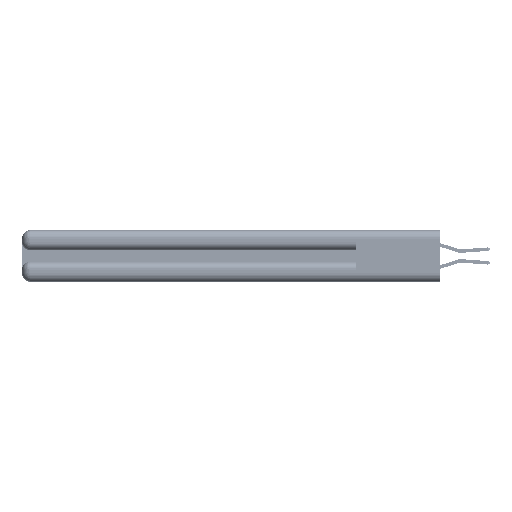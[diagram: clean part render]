
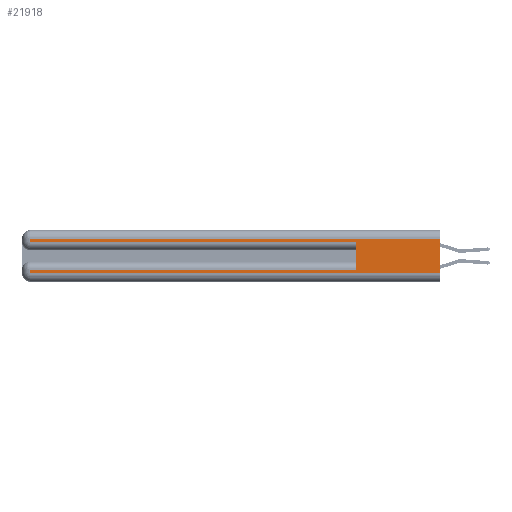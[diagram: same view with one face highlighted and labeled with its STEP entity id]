
A CAD part, left-side view. The second image highlights one B-rep face of the part: STEP entity #21918.
In plain terms, the highlighted planar face has unit normal (-1, 0, 0).
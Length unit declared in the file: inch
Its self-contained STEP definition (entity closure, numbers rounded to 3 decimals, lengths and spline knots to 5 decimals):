
#513 = DIRECTION ( 'NONE',  ( 0., 0., -1. ) ) ;
#689 = CARTESIAN_POINT ( 'NONE',  ( 0., 0., 0.31 ) ) ;
#1498 = ORIENTED_EDGE ( 'NONE', *, *, #36229, .F. ) ;
#2622 = VERTEX_POINT ( 'NONE', #35464 ) ;
#4131 = EDGE_CURVE ( 'NONE', #45053, #15400, #28205, .T. ) ;
#5082 = VERTEX_POINT ( 'NONE', #50191 ) ;
#5464 = VERTEX_POINT ( 'NONE', #32988 ) ;
#5556 = AXIS2_PLACEMENT_3D ( 'NONE', #40355, #47972, #39653 ) ;
#7135 = VECTOR ( 'NONE', #33044, 39.37008 ) ;
#7574 = LINE ( 'NONE', #22508, #49438 ) ;
#7947 = CARTESIAN_POINT ( 'NONE',  ( 0., 0.6, 0.145 ) ) ;
#11668 = PLANE ( 'NONE',  #5556 ) ;
#12085 = CARTESIAN_POINT ( 'NONE',  ( 0., 0., 0.37 ) ) ;
#12263 = VERTEX_POINT ( 'NONE', #689 ) ;
#14483 = DIRECTION ( 'NONE',  ( 0., 1., 0. ) ) ;
#15284 = ORIENTED_EDGE ( 'NONE', *, *, #4131, .T. ) ;
#15400 = VERTEX_POINT ( 'NONE', #36841 ) ;
#15733 = DIRECTION ( 'NONE',  ( 0., 0., 1. ) ) ;
#16863 = ORIENTED_EDGE ( 'NONE', *, *, #29857, .T. ) ;
#19914 = VERTEX_POINT ( 'NONE', #24833 ) ;
#20350 = VECTOR ( 'NONE', #49502, 39.37008 ) ;
#20726 = ORIENTED_EDGE ( 'NONE', *, *, #31548, .F. ) ;
#20822 = ORIENTED_EDGE ( 'NONE', *, *, #29239, .T. ) ;
#21685 = CARTESIAN_POINT ( 'NONE',  ( 0., 2.94, 0.31 ) ) ;
#21918 = ADVANCED_FACE ( 'NONE', ( #40342 ), #11668, .F. ) ;
#22508 = CARTESIAN_POINT ( 'NONE',  ( 0., 0., 0.31 ) ) ;
#22517 = VECTOR ( 'NONE', #45650, 39.37008 ) ;
#22911 = LINE ( 'NONE', #33758, #20350 ) ;
#24630 = LINE ( 'NONE', #12085, #37282 ) ;
#24833 = CARTESIAN_POINT ( 'NONE',  ( 0., 2.94, 0.085 ) ) ;
#25293 = CARTESIAN_POINT ( 'NONE',  ( 0., 2.94, 0.37 ) ) ;
#27809 = LINE ( 'NONE', #7947, #48065 ) ;
#27908 = DIRECTION ( 'NONE',  ( 0., 1., 0. ) ) ;
#28205 = LINE ( 'NONE', #25293, #22517 ) ;
#28743 = LINE ( 'NONE', #36910, #7135 ) ;
#29000 = EDGE_CURVE ( 'NONE', #2622, #5082, #22911, .T. ) ;
#29239 = EDGE_CURVE ( 'NONE', #19914, #2622, #33661, .T. ) ;
#29386 = ORIENTED_EDGE ( 'NONE', *, *, #33042, .T. ) ;
#29857 = EDGE_CURVE ( 'NONE', #12263, #45053, #7574, .T. ) ;
#30494 = CARTESIAN_POINT ( 'NONE',  ( 0., 0.6, 0.285 ) ) ;
#31426 = CARTESIAN_POINT ( 'NONE',  ( 0., 2.94, 0.37 ) ) ;
#31548 = EDGE_CURVE ( 'NONE', #5464, #40568, #27809, .T. ) ;
#32988 = CARTESIAN_POINT ( 'NONE',  ( 0., 0.6, 0.085 ) ) ;
#33042 = EDGE_CURVE ( 'NONE', #15400, #40568, #28743, .T. ) ;
#33044 = DIRECTION ( 'NONE',  ( 0., -1., 0. ) ) ;
#33180 = VECTOR ( 'NONE', #27908, 39.37008 ) ;
#33661 = LINE ( 'NONE', #31426, #48817 ) ;
#33758 = CARTESIAN_POINT ( 'NONE',  ( 0., 0., 0.06 ) ) ;
#35464 = CARTESIAN_POINT ( 'NONE',  ( 0., 2.94, 0.06 ) ) ;
#36229 = EDGE_CURVE ( 'NONE', #12263, #5082, #24630, .T. ) ;
#36841 = CARTESIAN_POINT ( 'NONE',  ( 0., 2.94, 0.285 ) ) ;
#36910 = CARTESIAN_POINT ( 'NONE',  ( 0., 0., 0.285 ) ) ;
#37157 = EDGE_LOOP ( 'NONE', ( #1498, #16863, #15284, #29386, #20726, #50731, #20822, #42375 ) ) ;
#37282 = VECTOR ( 'NONE', #513, 39.37008 ) ;
#39497 = LINE ( 'NONE', #40452, #33180 ) ;
#39653 = DIRECTION ( 'NONE',  ( 0., 0., -1. ) ) ;
#40342 = FACE_OUTER_BOUND ( 'NONE', #37157, .T. ) ;
#40355 = CARTESIAN_POINT ( 'NONE',  ( 0., 0., 0.37 ) ) ;
#40452 = CARTESIAN_POINT ( 'NONE',  ( 0., 0., 0.085 ) ) ;
#40568 = VERTEX_POINT ( 'NONE', #30494 ) ;
#42375 = ORIENTED_EDGE ( 'NONE', *, *, #29000, .T. ) ;
#43762 = DIRECTION ( 'NONE',  ( 0., 0., -1. ) ) ;
#45053 = VERTEX_POINT ( 'NONE', #21685 ) ;
#45650 = DIRECTION ( 'NONE',  ( 0., 0., -1. ) ) ;
#47878 = EDGE_CURVE ( 'NONE', #5464, #19914, #39497, .T. ) ;
#47972 = DIRECTION ( 'NONE',  ( 1., 0., 0. ) ) ;
#48065 = VECTOR ( 'NONE', #15733, 39.37008 ) ;
#48817 = VECTOR ( 'NONE', #43762, 39.37008 ) ;
#49438 = VECTOR ( 'NONE', #14483, 39.37008 ) ;
#49502 = DIRECTION ( 'NONE',  ( 0., -1., 0. ) ) ;
#50191 = CARTESIAN_POINT ( 'NONE',  ( 0., 0., 0.06 ) ) ;
#50731 = ORIENTED_EDGE ( 'NONE', *, *, #47878, .T. ) ;
